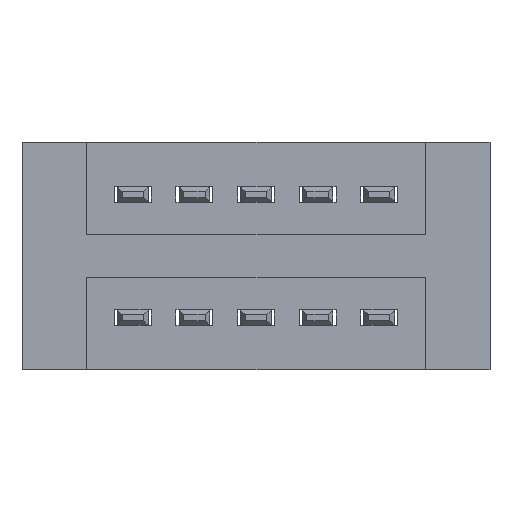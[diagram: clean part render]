
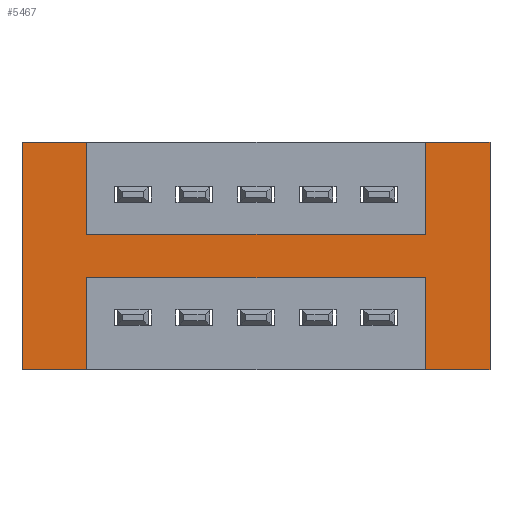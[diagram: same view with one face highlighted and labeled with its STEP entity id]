
A CAD part, front view. The second image highlights one B-rep face of the part: STEP entity #5467.
In plain terms, the highlighted planar face has unit normal (0, -1, 0).
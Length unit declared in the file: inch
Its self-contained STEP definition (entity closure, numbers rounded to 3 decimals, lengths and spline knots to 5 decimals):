
#153 = CARTESIAN_POINT ( 'NONE',  ( 0., 0., -0.37 ) ) ;
#157 = LINE ( 'NONE', #479, #5974 ) ;
#235 = FACE_OUTER_BOUND ( 'NONE', #1433, .T. ) ;
#260 = ORIENTED_EDGE ( 'NONE', *, *, #7130, .T. ) ;
#266 = LINE ( 'NONE', #153, #5054 ) ;
#408 = DIRECTION ( 'NONE',  ( 0., 0., -1. ) ) ;
#479 = CARTESIAN_POINT ( 'NONE',  ( 0.3925, 0., -0.15 ) ) ;
#488 = DIRECTION ( 'NONE',  ( 0., 0., -1. ) ) ;
#542 = CARTESIAN_POINT ( 'NONE',  ( 1.0475, 0., -0.37 ) ) ;
#678 = VERTEX_POINT ( 'NONE', #7666 ) ;
#787 = LINE ( 'NONE', #958, #8360 ) ;
#803 = CARTESIAN_POINT ( 'NONE',  ( 0.2875, 0., -0.37 ) ) ;
#882 = DIRECTION ( 'NONE',  ( 0., 0., 1. ) ) ;
#958 = CARTESIAN_POINT ( 'NONE',  ( 0., 0., -0.37 ) ) ;
#1007 = DIRECTION ( 'NONE',  ( -1., 0., 0. ) ) ;
#1128 = VECTOR ( 'NONE', #3623, 39.37008 ) ;
#1168 = EDGE_CURVE ( 'NONE', #3484, #8020, #7096, .T. ) ;
#1277 = VERTEX_POINT ( 'NONE', #542 ) ;
#1332 = DIRECTION ( 'NONE',  ( 0., 0., 1. ) ) ;
#1400 = VECTOR ( 'NONE', #7154, 39.37008 ) ;
#1420 = LINE ( 'NONE', #2294, #7366 ) ;
#1423 = LINE ( 'NONE', #2627, #3568 ) ;
#1433 = EDGE_LOOP ( 'NONE', ( #7633, #3628, #7485, #1497, #6014, #6290, #260, #2312, #4371, #7053, #8181, #5461 ) ) ;
#1480 = LINE ( 'NONE', #6211, #4732 ) ;
#1497 = ORIENTED_EDGE ( 'NONE', *, *, #3671, .F. ) ;
#1567 = EDGE_CURVE ( 'NONE', #1277, #3699, #6575, .T. ) ;
#1737 = CARTESIAN_POINT ( 'NONE',  ( 1.0475, 0., 0. ) ) ;
#1815 = DIRECTION ( 'NONE',  ( 1., 0., 0. ) ) ;
#2200 = EDGE_CURVE ( 'NONE', #678, #3858, #1420, .T. ) ;
#2294 = CARTESIAN_POINT ( 'NONE',  ( 0.3925, 0., -0.22 ) ) ;
#2310 = VERTEX_POINT ( 'NONE', #5360 ) ;
#2312 = ORIENTED_EDGE ( 'NONE', *, *, #2368, .F. ) ;
#2368 = EDGE_CURVE ( 'NONE', #4758, #8421, #787, .T. ) ;
#2542 = CARTESIAN_POINT ( 'NONE',  ( 0.9425, 0., -0.37 ) ) ;
#2627 = CARTESIAN_POINT ( 'NONE',  ( 0.9425, 0., -0.37 ) ) ;
#2791 = LINE ( 'NONE', #5691, #4517 ) ;
#3061 = CARTESIAN_POINT ( 'NONE',  ( 0.2875, 0., 0. ) ) ;
#3252 = EDGE_CURVE ( 'NONE', #2310, #3449, #6615, .T. ) ;
#3449 = VERTEX_POINT ( 'NONE', #5280 ) ;
#3484 = VERTEX_POINT ( 'NONE', #7922 ) ;
#3523 = CARTESIAN_POINT ( 'NONE',  ( 0., 0., -0.37 ) ) ;
#3568 = VECTOR ( 'NONE', #1332, 39.37008 ) ;
#3593 = VECTOR ( 'NONE', #3616, 39.37008 ) ;
#3616 = DIRECTION ( 'NONE',  ( 0., 0., -1. ) ) ;
#3623 = DIRECTION ( 'NONE',  ( 1., 0., 0. ) ) ;
#3628 = ORIENTED_EDGE ( 'NONE', *, *, #5684, .F. ) ;
#3671 = EDGE_CURVE ( 'NONE', #8020, #2310, #157, .T. ) ;
#3699 = VERTEX_POINT ( 'NONE', #1737 ) ;
#3858 = VERTEX_POINT ( 'NONE', #4351 ) ;
#4098 = LINE ( 'NONE', #5669, #3593 ) ;
#4124 = DIRECTION ( 'NONE',  ( 0., 0., -1. ) ) ;
#4215 = CARTESIAN_POINT ( 'NONE',  ( 0.3925, 0., -0.37 ) ) ;
#4351 = CARTESIAN_POINT ( 'NONE',  ( 0.3925, 0., -0.22 ) ) ;
#4371 = ORIENTED_EDGE ( 'NONE', *, *, #5130, .F. ) ;
#4514 = VECTOR ( 'NONE', #488, 39.37008 ) ;
#4517 = VECTOR ( 'NONE', #1815, 39.37008 ) ;
#4562 = CARTESIAN_POINT ( 'NONE',  ( 0.9425, 0., 0. ) ) ;
#4732 = VECTOR ( 'NONE', #408, 39.37008 ) ;
#4758 = VERTEX_POINT ( 'NONE', #4215 ) ;
#4805 = VECTOR ( 'NONE', #882, 39.37008 ) ;
#4871 = DIRECTION ( 'NONE',  ( -1., 0., 0. ) ) ;
#5029 = DIRECTION ( 'NONE',  ( 1., 0., 0. ) ) ;
#5054 = VECTOR ( 'NONE', #5273, 39.37008 ) ;
#5130 = EDGE_CURVE ( 'NONE', #3858, #4758, #1480, .T. ) ;
#5273 = DIRECTION ( 'NONE',  ( -1., 0., 0. ) ) ;
#5280 = CARTESIAN_POINT ( 'NONE',  ( 0.9425, 0., 0. ) ) ;
#5353 = DIRECTION ( 'NONE',  ( 0., -1., 0. ) ) ;
#5360 = CARTESIAN_POINT ( 'NONE',  ( 0.9425, 0., -0.15 ) ) ;
#5461 = ORIENTED_EDGE ( 'NONE', *, *, #8396, .F. ) ;
#5467 = ADVANCED_FACE ( 'NONE', ( #235 ), #7989, .T. ) ;
#5521 = AXIS2_PLACEMENT_3D ( 'NONE', #3523, #5353, #4124 ) ;
#5669 = CARTESIAN_POINT ( 'NONE',  ( 0.2875, 0., 0. ) ) ;
#5684 = EDGE_CURVE ( 'NONE', #3449, #3699, #2791, .T. ) ;
#5691 = CARTESIAN_POINT ( 'NONE',  ( 0., 0., 0. ) ) ;
#5974 = VECTOR ( 'NONE', #5029, 39.37008 ) ;
#6014 = ORIENTED_EDGE ( 'NONE', *, *, #1168, .F. ) ;
#6211 = CARTESIAN_POINT ( 'NONE',  ( 0.3925, 0., -0.37 ) ) ;
#6213 = CARTESIAN_POINT ( 'NONE',  ( 0., 0., 0. ) ) ;
#6290 = ORIENTED_EDGE ( 'NONE', *, *, #7903, .F. ) ;
#6575 = LINE ( 'NONE', #8057, #4805 ) ;
#6615 = LINE ( 'NONE', #4562, #1400 ) ;
#6968 = VERTEX_POINT ( 'NONE', #3061 ) ;
#7053 = ORIENTED_EDGE ( 'NONE', *, *, #2200, .F. ) ;
#7096 = LINE ( 'NONE', #8311, #4514 ) ;
#7130 = EDGE_CURVE ( 'NONE', #6968, #8421, #4098, .T. ) ;
#7154 = DIRECTION ( 'NONE',  ( 0., 0., 1. ) ) ;
#7366 = VECTOR ( 'NONE', #1007, 39.37008 ) ;
#7378 = LINE ( 'NONE', #6213, #1128 ) ;
#7485 = ORIENTED_EDGE ( 'NONE', *, *, #3252, .F. ) ;
#7633 = ORIENTED_EDGE ( 'NONE', *, *, #1567, .T. ) ;
#7666 = CARTESIAN_POINT ( 'NONE',  ( 0.9425, 0., -0.22 ) ) ;
#7750 = CARTESIAN_POINT ( 'NONE',  ( 0.3925, 0., -0.15 ) ) ;
#7903 = EDGE_CURVE ( 'NONE', #6968, #3484, #7378, .T. ) ;
#7922 = CARTESIAN_POINT ( 'NONE',  ( 0.3925, 0., 0. ) ) ;
#7989 = PLANE ( 'NONE',  #5521 ) ;
#8020 = VERTEX_POINT ( 'NONE', #7750 ) ;
#8057 = CARTESIAN_POINT ( 'NONE',  ( 1.0475, 0., 0. ) ) ;
#8156 = EDGE_CURVE ( 'NONE', #8187, #678, #1423, .T. ) ;
#8181 = ORIENTED_EDGE ( 'NONE', *, *, #8156, .F. ) ;
#8187 = VERTEX_POINT ( 'NONE', #2542 ) ;
#8311 = CARTESIAN_POINT ( 'NONE',  ( 0.3925, 0., 0. ) ) ;
#8360 = VECTOR ( 'NONE', #4871, 39.37008 ) ;
#8396 = EDGE_CURVE ( 'NONE', #1277, #8187, #266, .T. ) ;
#8421 = VERTEX_POINT ( 'NONE', #803 ) ;
